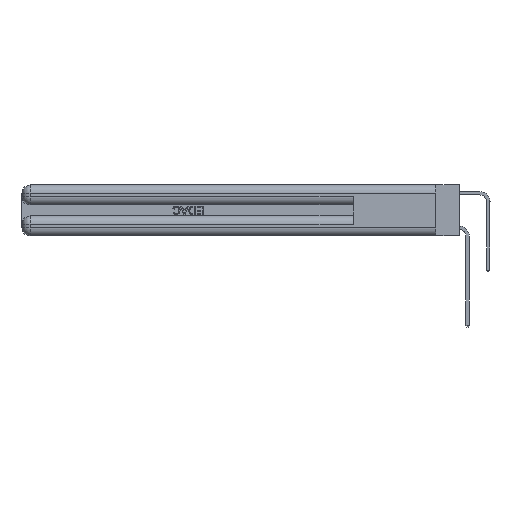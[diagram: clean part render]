
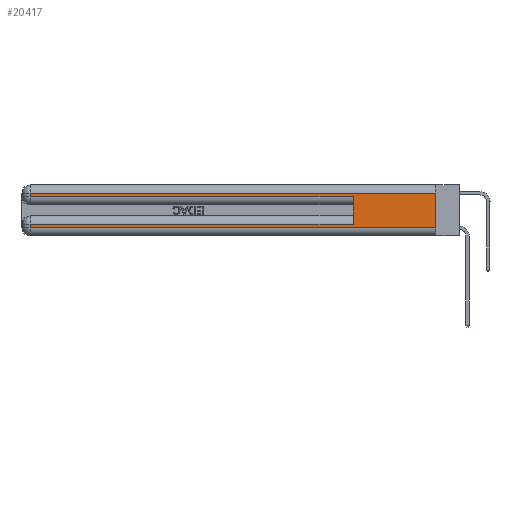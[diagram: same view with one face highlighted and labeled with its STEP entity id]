
A CAD part, left-side view. The second image highlights one B-rep face of the part: STEP entity #20417.
In plain terms, the highlighted planar face has unit normal (-1, 0, 0).
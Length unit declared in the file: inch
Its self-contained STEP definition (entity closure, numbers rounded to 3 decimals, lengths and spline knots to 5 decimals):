
#484 = VECTOR ( 'NONE', #21506, 39.37008 ) ;
#948 = CARTESIAN_POINT ( 'NONE',  ( 0., 0.6, 0.285 ) ) ;
#2003 = VECTOR ( 'NONE', #13696, 39.37008 ) ;
#3196 = DIRECTION ( 'NONE',  ( 0., 0., -1. ) ) ;
#3410 = CARTESIAN_POINT ( 'NONE',  ( 0., 0., 0.06 ) ) ;
#3998 = LINE ( 'NONE', #29261, #9251 ) ;
#4764 = ORIENTED_EDGE ( 'NONE', *, *, #5679, .T. ) ;
#4887 = EDGE_CURVE ( 'NONE', #27798, #18339, #14830, .T. ) ;
#4908 = DIRECTION ( 'NONE',  ( 0., -1., 0. ) ) ;
#5206 = VECTOR ( 'NONE', #30082, 39.37008 ) ;
#5679 = EDGE_CURVE ( 'NONE', #27798, #33365, #13296, .T. ) ;
#5775 = CARTESIAN_POINT ( 'NONE',  ( 0., 0., 0.37 ) ) ;
#6107 = EDGE_CURVE ( 'NONE', #25451, #24290, #12465, .T. ) ;
#6434 = CARTESIAN_POINT ( 'NONE',  ( 0., 0.6, 0.085 ) ) ;
#6628 = DIRECTION ( 'NONE',  ( 0., 0., -1. ) ) ;
#7409 = LINE ( 'NONE', #3410, #484 ) ;
#7506 = CARTESIAN_POINT ( 'NONE',  ( 0., 0., 0.37 ) ) ;
#7998 = ORIENTED_EDGE ( 'NONE', *, *, #4887, .F. ) ;
#9251 = VECTOR ( 'NONE', #13975, 39.37008 ) ;
#9252 = ORIENTED_EDGE ( 'NONE', *, *, #18412, .T. ) ;
#10058 = LINE ( 'NONE', #11968, #5206 ) ;
#10495 = ORIENTED_EDGE ( 'NONE', *, *, #28395, .T. ) ;
#10718 = CARTESIAN_POINT ( 'NONE',  ( 0., 2.94, 0.285 ) ) ;
#10955 = CARTESIAN_POINT ( 'NONE',  ( 0., 2.94, 0.085 ) ) ;
#10999 = CARTESIAN_POINT ( 'NONE',  ( 0., 0., 0.31 ) ) ;
#11580 = DIRECTION ( 'NONE',  ( 0., 0., 1. ) ) ;
#11815 = LINE ( 'NONE', #22024, #23147 ) ;
#11968 = CARTESIAN_POINT ( 'NONE',  ( 0., 0., 0.085 ) ) ;
#12152 = EDGE_CURVE ( 'NONE', #15307, #18339, #7409, .T. ) ;
#12192 = VERTEX_POINT ( 'NONE', #6434 ) ;
#12465 = LINE ( 'NONE', #15389, #16951 ) ;
#13296 = LINE ( 'NONE', #10999, #2003 ) ;
#13696 = DIRECTION ( 'NONE',  ( 0., 1., 0. ) ) ;
#13923 = EDGE_CURVE ( 'NONE', #12192, #24290, #30372, .T. ) ;
#13975 = DIRECTION ( 'NONE',  ( 0., 0., -1. ) ) ;
#14830 = LINE ( 'NONE', #7506, #18047 ) ;
#15307 = VERTEX_POINT ( 'NONE', #27796 ) ;
#15389 = CARTESIAN_POINT ( 'NONE',  ( 0., 0., 0.285 ) ) ;
#16951 = VECTOR ( 'NONE', #4908, 39.37008 ) ;
#17325 = ORIENTED_EDGE ( 'NONE', *, *, #12152, .T. ) ;
#17564 = ORIENTED_EDGE ( 'NONE', *, *, #13923, .F. ) ;
#18047 = VECTOR ( 'NONE', #18592, 39.37008 ) ;
#18339 = VERTEX_POINT ( 'NONE', #21617 ) ;
#18412 = EDGE_CURVE ( 'NONE', #12192, #22296, #10058, .T. ) ;
#18592 = DIRECTION ( 'NONE',  ( 0., 0., -1. ) ) ;
#19256 = FACE_OUTER_BOUND ( 'NONE', #30947, .T. ) ;
#20384 = AXIS2_PLACEMENT_3D ( 'NONE', #5775, #31678, #3196 ) ;
#20417 = ADVANCED_FACE ( 'NONE', ( #19256 ), #29072, .F. ) ;
#21506 = DIRECTION ( 'NONE',  ( 0., -1., 0. ) ) ;
#21617 = CARTESIAN_POINT ( 'NONE',  ( 0., 0., 0.06 ) ) ;
#22024 = CARTESIAN_POINT ( 'NONE',  ( 0., 2.94, 0.37 ) ) ;
#22296 = VERTEX_POINT ( 'NONE', #10955 ) ;
#23147 = VECTOR ( 'NONE', #6628, 39.37008 ) ;
#23322 = ORIENTED_EDGE ( 'NONE', *, *, #6107, .T. ) ;
#24290 = VERTEX_POINT ( 'NONE', #948 ) ;
#24515 = CARTESIAN_POINT ( 'NONE',  ( 0., 0.6, 0.145 ) ) ;
#25451 = VERTEX_POINT ( 'NONE', #10718 ) ;
#27502 = CARTESIAN_POINT ( 'NONE',  ( 0., 0., 0.31 ) ) ;
#27796 = CARTESIAN_POINT ( 'NONE',  ( 0., 2.94, 0.06 ) ) ;
#27798 = VERTEX_POINT ( 'NONE', #27502 ) ;
#28395 = EDGE_CURVE ( 'NONE', #22296, #15307, #11815, .T. ) ;
#29072 = PLANE ( 'NONE',  #20384 ) ;
#29261 = CARTESIAN_POINT ( 'NONE',  ( 0., 2.94, 0.37 ) ) ;
#30082 = DIRECTION ( 'NONE',  ( 0., 1., 0. ) ) ;
#30372 = LINE ( 'NONE', #24515, #31583 ) ;
#30947 = EDGE_LOOP ( 'NONE', ( #7998, #4764, #32907, #23322, #17564, #9252, #10495, #17325 ) ) ;
#31583 = VECTOR ( 'NONE', #11580, 39.37008 ) ;
#31635 = EDGE_CURVE ( 'NONE', #33365, #25451, #3998, .T. ) ;
#31678 = DIRECTION ( 'NONE',  ( 1., 0., 0. ) ) ;
#32907 = ORIENTED_EDGE ( 'NONE', *, *, #31635, .T. ) ;
#32977 = CARTESIAN_POINT ( 'NONE',  ( 0., 2.94, 0.31 ) ) ;
#33365 = VERTEX_POINT ( 'NONE', #32977 ) ;
